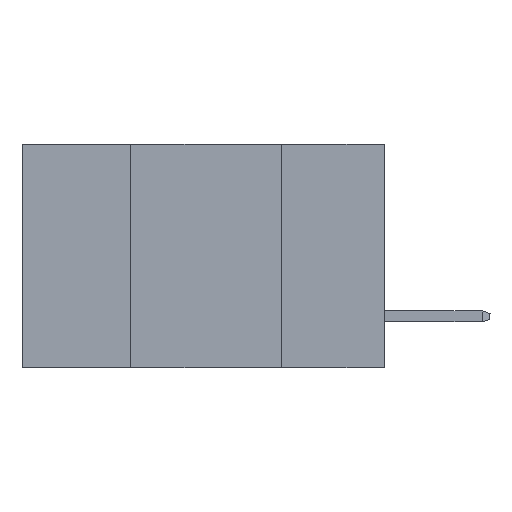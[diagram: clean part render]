
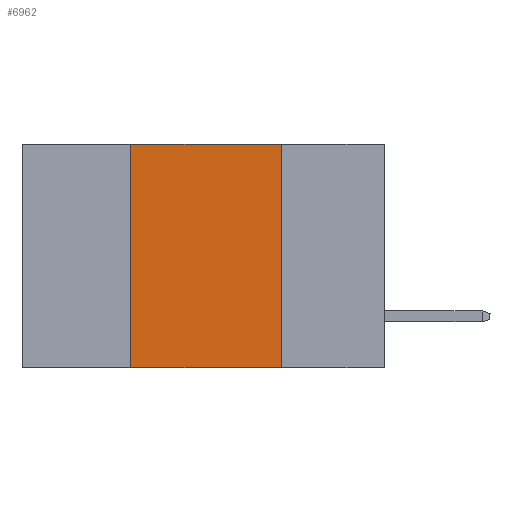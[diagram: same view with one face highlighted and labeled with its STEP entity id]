
A CAD part, left-side view. The second image highlights one B-rep face of the part: STEP entity #6962.
In plain terms, the highlighted planar face has unit normal (-1, 0, 0).
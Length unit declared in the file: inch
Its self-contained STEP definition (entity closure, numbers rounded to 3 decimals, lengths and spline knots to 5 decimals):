
#450 = VECTOR ( 'NONE', #10815, 39.37008 ) ;
#1069 = EDGE_CURVE ( 'NONE', #12425, #16330, #3710, .T. ) ;
#1985 = CARTESIAN_POINT ( 'NONE',  ( 0., 0.6, 0. ) ) ;
#2262 = ORIENTED_EDGE ( 'NONE', *, *, #1069, .F. ) ;
#2711 = CARTESIAN_POINT ( 'NONE',  ( 0., 0.42, -0.37 ) ) ;
#2938 = ORIENTED_EDGE ( 'NONE', *, *, #4347, .F. ) ;
#3710 = LINE ( 'NONE', #17889, #4199 ) ;
#3819 = CARTESIAN_POINT ( 'NONE',  ( 0., 0.17, 0. ) ) ;
#4199 = VECTOR ( 'NONE', #15139, 39.37008 ) ;
#4347 = EDGE_CURVE ( 'NONE', #17634, #12425, #5210, .T. ) ;
#4631 = VERTEX_POINT ( 'NONE', #12768 ) ;
#4916 = PLANE ( 'NONE',  #16651 ) ;
#5210 = LINE ( 'NONE', #1985, #450 ) ;
#6111 = CARTESIAN_POINT ( 'NONE',  ( 0., 0.6, -0.37 ) ) ;
#6717 = ORIENTED_EDGE ( 'NONE', *, *, #17310, .T. ) ;
#6962 = ADVANCED_FACE ( 'NONE', ( #13485 ), #4916, .F. ) ;
#7024 = CARTESIAN_POINT ( 'NONE',  ( 0., 0.42, 0. ) ) ;
#8328 = DIRECTION ( 'NONE',  ( 0., 0., 1. ) ) ;
#8954 = DIRECTION ( 'NONE',  ( 0., -1., 0. ) ) ;
#9331 = DIRECTION ( 'NONE',  ( 0., 0., -1. ) ) ;
#9759 = EDGE_LOOP ( 'NONE', ( #2262, #2938, #14861, #6717 ) ) ;
#10815 = DIRECTION ( 'NONE',  ( 0., -1., 0. ) ) ;
#11071 = CARTESIAN_POINT ( 'NONE',  ( 0., 0.17, -0.37 ) ) ;
#11808 = LINE ( 'NONE', #6111, #13627 ) ;
#12425 = VERTEX_POINT ( 'NONE', #3819 ) ;
#12613 = EDGE_CURVE ( 'NONE', #4631, #17634, #17006, .T. ) ;
#12768 = CARTESIAN_POINT ( 'NONE',  ( 0., 0.42, -0.37 ) ) ;
#13394 = DIRECTION ( 'NONE',  ( 1., 0., 0. ) ) ;
#13485 = FACE_OUTER_BOUND ( 'NONE', #9759, .T. ) ;
#13627 = VECTOR ( 'NONE', #8954, 39.37008 ) ;
#13669 = CARTESIAN_POINT ( 'NONE',  ( 0., 0.6, 0. ) ) ;
#14861 = ORIENTED_EDGE ( 'NONE', *, *, #12613, .F. ) ;
#15139 = DIRECTION ( 'NONE',  ( 0., 0., -1. ) ) ;
#16330 = VERTEX_POINT ( 'NONE', #11071 ) ;
#16499 = VECTOR ( 'NONE', #8328, 39.37008 ) ;
#16651 = AXIS2_PLACEMENT_3D ( 'NONE', #13669, #13394, #9331 ) ;
#17006 = LINE ( 'NONE', #2711, #16499 ) ;
#17310 = EDGE_CURVE ( 'NONE', #4631, #16330, #11808, .T. ) ;
#17634 = VERTEX_POINT ( 'NONE', #7024 ) ;
#17889 = CARTESIAN_POINT ( 'NONE',  ( 0., 0.17, -0.37 ) ) ;
